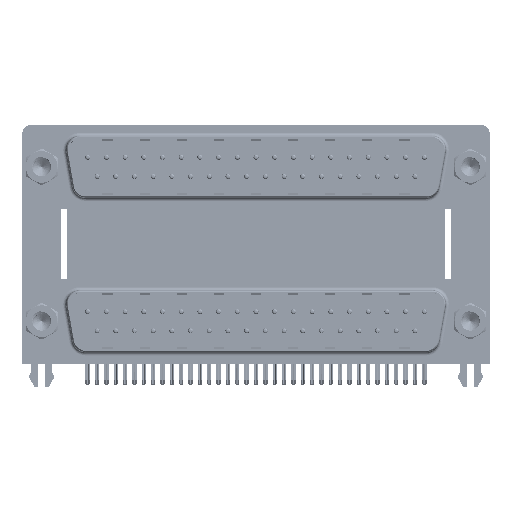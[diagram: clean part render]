
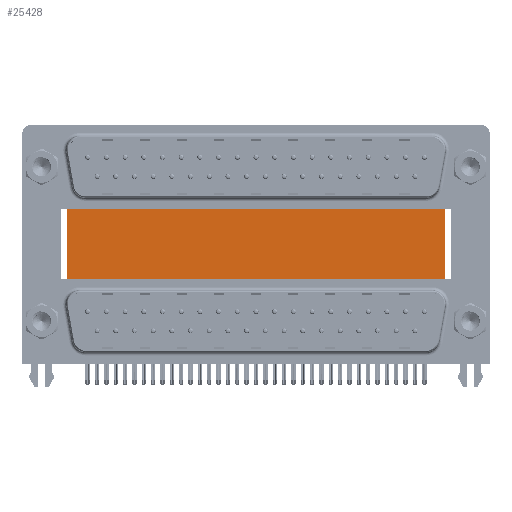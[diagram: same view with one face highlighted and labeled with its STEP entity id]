
A CAD part, top view. The second image highlights one B-rep face of the part: STEP entity #25428.
In plain terms, the highlighted planar face has unit normal (0, 0, 1).
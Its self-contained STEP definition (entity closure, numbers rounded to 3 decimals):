
#413 = VERTEX_POINT ( 'NONE', #37382 ) ;
#577 = VECTOR ( 'NONE', #5265, 1000. ) ;
#828 = CARTESIAN_POINT ( 'NONE',  ( 3.79, 16.585, -12. ) ) ;
#918 = LINE ( 'NONE', #18931, #28300 ) ;
#2958 = ORIENTED_EDGE ( 'NONE', *, *, #3436, .F. ) ;
#3044 = DIRECTION ( 'NONE',  ( 1., 0., 0. ) ) ;
#3436 = EDGE_CURVE ( 'NONE', #413, #48116, #15141, .T. ) ;
#4787 = EDGE_CURVE ( 'NONE', #35246, #48116, #42862, .T. ) ;
#5265 = DIRECTION ( 'NONE',  ( 1., 0., 0. ) ) ;
#9494 = DIRECTION ( 'NONE',  ( 0., -1., 0. ) ) ;
#10224 = CARTESIAN_POINT ( 'NONE',  ( 3.79, -3.735, -12. ) ) ;
#14561 = CARTESIAN_POINT ( 'NONE',  ( 59.71, -3.735, -12. ) ) ;
#15141 = LINE ( 'NONE', #55215, #58126 ) ;
#16079 = ORIENTED_EDGE ( 'NONE', *, *, #48501, .T. ) ;
#18931 = CARTESIAN_POINT ( 'NONE',  ( 3.79, 16.585, -12. ) ) ;
#20394 = VERTEX_POINT ( 'NONE', #30732 ) ;
#24025 = AXIS2_PLACEMENT_3D ( 'NONE', #51677, #29541, #33951 ) ;
#24543 = FACE_OUTER_BOUND ( 'NONE', #40016, .T. ) ;
#25428 = ADVANCED_FACE ( 'NONE', ( #24543 ), #56684, .F. ) ;
#27901 = VECTOR ( 'NONE', #3044, 1000. ) ;
#28300 = VECTOR ( 'NONE', #9494, 1000. ) ;
#28957 = ORIENTED_EDGE ( 'NONE', *, *, #4787, .T. ) ;
#29541 = DIRECTION ( 'NONE',  ( 0., 0., -1. ) ) ;
#30732 = CARTESIAN_POINT ( 'NONE',  ( 3.79, 16.585, -12. ) ) ;
#33951 = DIRECTION ( 'NONE',  ( -1., 0., 0. ) ) ;
#35246 = VERTEX_POINT ( 'NONE', #10224 ) ;
#36948 = ORIENTED_EDGE ( 'NONE', *, *, #38263, .F. ) ;
#37382 = CARTESIAN_POINT ( 'NONE',  ( 59.71, 16.585, -12. ) ) ;
#37673 = LINE ( 'NONE', #828, #577 ) ;
#38263 = EDGE_CURVE ( 'NONE', #20394, #413, #37673, .T. ) ;
#40016 = EDGE_LOOP ( 'NONE', ( #28957, #2958, #36948, #16079 ) ) ;
#41670 = DIRECTION ( 'NONE',  ( 0., -1., 0. ) ) ;
#42862 = LINE ( 'NONE', #43458, #27901 ) ;
#43458 = CARTESIAN_POINT ( 'NONE',  ( 3.79, -3.735, -12. ) ) ;
#48116 = VERTEX_POINT ( 'NONE', #14561 ) ;
#48501 = EDGE_CURVE ( 'NONE', #20394, #35246, #918, .T. ) ;
#51677 = CARTESIAN_POINT ( 'NONE',  ( 3.79, 16.585, -12. ) ) ;
#55215 = CARTESIAN_POINT ( 'NONE',  ( 59.71, 16.585, -12. ) ) ;
#56684 = PLANE ( 'NONE',  #24025 ) ;
#58126 = VECTOR ( 'NONE', #41670, 1000. ) ;
